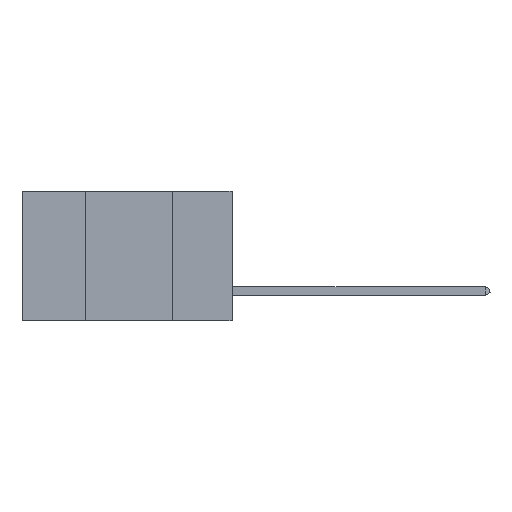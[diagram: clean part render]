
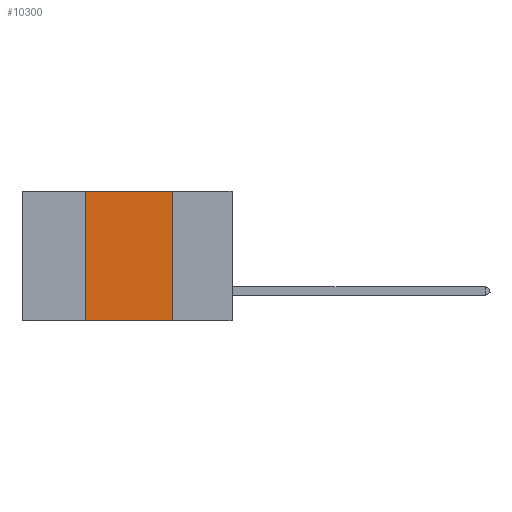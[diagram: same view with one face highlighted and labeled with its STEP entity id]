
A CAD part, left-side view. The second image highlights one B-rep face of the part: STEP entity #10300.
In plain terms, the highlighted planar face has unit normal (-1, 0, 0).
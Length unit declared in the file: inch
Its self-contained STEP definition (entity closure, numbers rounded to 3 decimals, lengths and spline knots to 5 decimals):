
#1059 = CARTESIAN_POINT ( 'NONE',  ( 0., 0.17, -0.37 ) ) ;
#1101 = DIRECTION ( 'NONE',  ( 1., 0., 0. ) ) ;
#1219 = EDGE_CURVE ( 'NONE', #12999, #1793, #12990, .T. ) ;
#1268 = CARTESIAN_POINT ( 'NONE',  ( 0., 0.42, 0. ) ) ;
#1326 = CARTESIAN_POINT ( 'NONE',  ( 0., 0.6, -0.37 ) ) ;
#1793 = VERTEX_POINT ( 'NONE', #2098 ) ;
#2098 = CARTESIAN_POINT ( 'NONE',  ( 0., 0.17, 0. ) ) ;
#2380 = VECTOR ( 'NONE', #12840, 39.37008 ) ;
#2478 = EDGE_CURVE ( 'NONE', #15935, #6677, #11605, .T. ) ;
#3896 = EDGE_LOOP ( 'NONE', ( #11999, #13277, #19827, #11793 ) ) ;
#4295 = FACE_OUTER_BOUND ( 'NONE', #3896, .T. ) ;
#4448 = CARTESIAN_POINT ( 'NONE',  ( 0., 0.6, 0. ) ) ;
#4556 = LINE ( 'NONE', #19652, #17363 ) ;
#6484 = DIRECTION ( 'NONE',  ( 0., -1., 0. ) ) ;
#6602 = AXIS2_PLACEMENT_3D ( 'NONE', #4448, #1101, #14462 ) ;
#6677 = VERTEX_POINT ( 'NONE', #1059 ) ;
#7958 = VECTOR ( 'NONE', #19909, 39.37008 ) ;
#8092 = CARTESIAN_POINT ( 'NONE',  ( 0., 0.42, -0.37 ) ) ;
#8320 = CARTESIAN_POINT ( 'NONE',  ( 0., 0.6, 0. ) ) ;
#8810 = EDGE_CURVE ( 'NONE', #1793, #6677, #4556, .T. ) ;
#10300 = ADVANCED_FACE ( 'NONE', ( #4295 ), #16138, .F. ) ;
#11605 = LINE ( 'NONE', #1326, #7958 ) ;
#11793 = ORIENTED_EDGE ( 'NONE', *, *, #2478, .T. ) ;
#11999 = ORIENTED_EDGE ( 'NONE', *, *, #8810, .F. ) ;
#12821 = EDGE_CURVE ( 'NONE', #15935, #12999, #15717, .T. ) ;
#12840 = DIRECTION ( 'NONE',  ( 0., 0., 1. ) ) ;
#12990 = LINE ( 'NONE', #8320, #20827 ) ;
#12999 = VERTEX_POINT ( 'NONE', #16690 ) ;
#13277 = ORIENTED_EDGE ( 'NONE', *, *, #1219, .F. ) ;
#14462 = DIRECTION ( 'NONE',  ( 0., 0., -1. ) ) ;
#15717 = LINE ( 'NONE', #1268, #2380 ) ;
#15935 = VERTEX_POINT ( 'NONE', #8092 ) ;
#16138 = PLANE ( 'NONE',  #6602 ) ;
#16690 = CARTESIAN_POINT ( 'NONE',  ( 0., 0.42, 0. ) ) ;
#17363 = VECTOR ( 'NONE', #21325, 39.37008 ) ;
#19652 = CARTESIAN_POINT ( 'NONE',  ( 0., 0.17, 0. ) ) ;
#19827 = ORIENTED_EDGE ( 'NONE', *, *, #12821, .F. ) ;
#19909 = DIRECTION ( 'NONE',  ( 0., -1., 0. ) ) ;
#20827 = VECTOR ( 'NONE', #6484, 39.37008 ) ;
#21325 = DIRECTION ( 'NONE',  ( 0., 0., -1. ) ) ;
